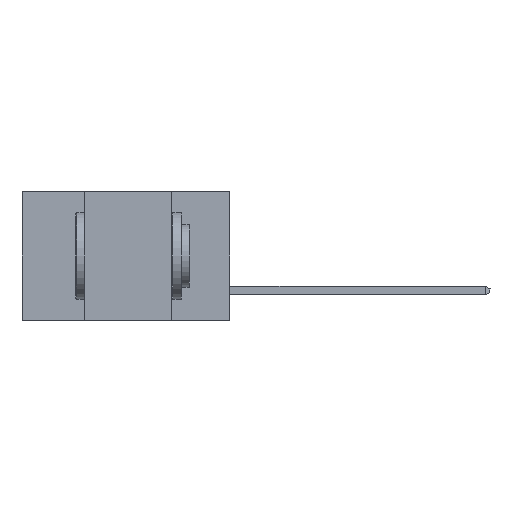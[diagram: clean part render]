
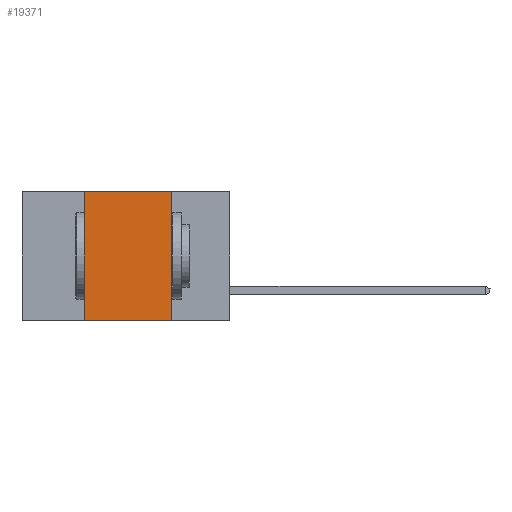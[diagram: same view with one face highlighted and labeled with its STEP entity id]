
A CAD part, left-side view. The second image highlights one B-rep face of the part: STEP entity #19371.
In plain terms, the highlighted planar face has unit normal (-1, 0, 0).
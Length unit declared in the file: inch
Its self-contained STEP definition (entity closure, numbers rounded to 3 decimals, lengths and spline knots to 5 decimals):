
#37 = VERTEX_POINT ( 'NONE', #5498 ) ;
#267 = VECTOR ( 'NONE', #6078, 39.37008 ) ;
#535 = DIRECTION ( 'NONE',  ( 0., 0., -1. ) ) ;
#685 = CARTESIAN_POINT ( 'NONE',  ( 0., 0.17, 0. ) ) ;
#1513 = DIRECTION ( 'NONE',  ( 1., 0., 0. ) ) ;
#2148 = EDGE_CURVE ( 'NONE', #10469, #37, #12921, .T. ) ;
#2797 = VERTEX_POINT ( 'NONE', #685 ) ;
#2963 = EDGE_CURVE ( 'NONE', #13446, #2797, #15964, .T. ) ;
#3346 = CARTESIAN_POINT ( 'NONE',  ( 0., 0.42, -0.37 ) ) ;
#4634 = VECTOR ( 'NONE', #19599, 39.37008 ) ;
#5498 = CARTESIAN_POINT ( 'NONE',  ( 0., 0.17, -0.37 ) ) ;
#5772 = ORIENTED_EDGE ( 'NONE', *, *, #2148, .T. ) ;
#6016 = ORIENTED_EDGE ( 'NONE', *, *, #16293, .F. ) ;
#6075 = VECTOR ( 'NONE', #535, 39.37008 ) ;
#6078 = DIRECTION ( 'NONE',  ( 0., -1., 0. ) ) ;
#6286 = CARTESIAN_POINT ( 'NONE',  ( 0., 0.42, -0.37 ) ) ;
#7106 = ORIENTED_EDGE ( 'NONE', *, *, #11620, .F. ) ;
#7901 = CARTESIAN_POINT ( 'NONE',  ( 0., 0.42, 0. ) ) ;
#7976 = CARTESIAN_POINT ( 'NONE',  ( 0., 0.6, 0. ) ) ;
#9504 = LINE ( 'NONE', #6286, #9809 ) ;
#9767 = CARTESIAN_POINT ( 'NONE',  ( 0., 0.6, -0.37 ) ) ;
#9809 = VECTOR ( 'NONE', #20756, 39.37008 ) ;
#10469 = VERTEX_POINT ( 'NONE', #3346 ) ;
#11588 = LINE ( 'NONE', #18062, #6075 ) ;
#11620 = EDGE_CURVE ( 'NONE', #2797, #37, #11588, .T. ) ;
#11895 = AXIS2_PLACEMENT_3D ( 'NONE', #7976, #1513, #20946 ) ;
#12921 = LINE ( 'NONE', #9767, #4634 ) ;
#13446 = VERTEX_POINT ( 'NONE', #7901 ) ;
#15399 = ORIENTED_EDGE ( 'NONE', *, *, #2963, .F. ) ;
#15846 = PLANE ( 'NONE',  #11895 ) ;
#15964 = LINE ( 'NONE', #18941, #267 ) ;
#16293 = EDGE_CURVE ( 'NONE', #10469, #13446, #9504, .T. ) ;
#18062 = CARTESIAN_POINT ( 'NONE',  ( 0., 0.17, -0.37 ) ) ;
#18941 = CARTESIAN_POINT ( 'NONE',  ( 0., 0.6, 0. ) ) ;
#19371 = ADVANCED_FACE ( 'NONE', ( #20748 ), #15846, .F. ) ;
#19599 = DIRECTION ( 'NONE',  ( 0., -1., 0. ) ) ;
#20589 = EDGE_LOOP ( 'NONE', ( #7106, #15399, #6016, #5772 ) ) ;
#20748 = FACE_OUTER_BOUND ( 'NONE', #20589, .T. ) ;
#20756 = DIRECTION ( 'NONE',  ( 0., 0., 1. ) ) ;
#20946 = DIRECTION ( 'NONE',  ( 0., 0., -1. ) ) ;
